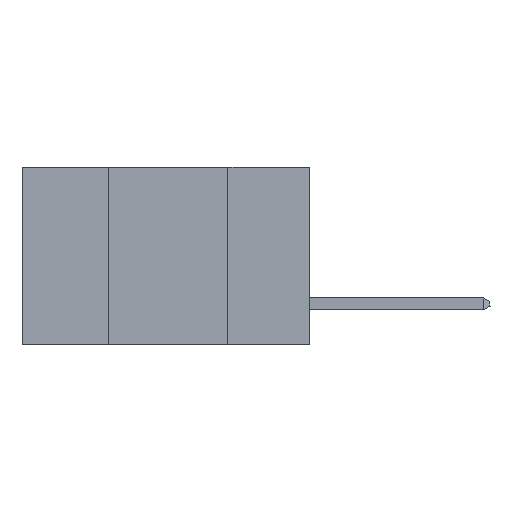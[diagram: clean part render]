
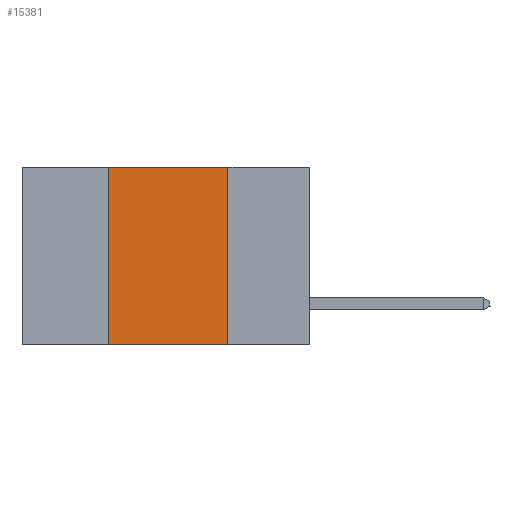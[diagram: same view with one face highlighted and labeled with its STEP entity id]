
A CAD part, left-side view. The second image highlights one B-rep face of the part: STEP entity #15381.
In plain terms, the highlighted planar face has unit normal (-1, 0, 0).
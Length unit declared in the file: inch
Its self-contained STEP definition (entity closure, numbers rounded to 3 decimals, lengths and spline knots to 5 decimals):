
#350 = FACE_OUTER_BOUND ( 'NONE', #20700, .T. ) ;
#760 = CARTESIAN_POINT ( 'NONE',  ( 0., 0.6, 0. ) ) ;
#2174 = ORIENTED_EDGE ( 'NONE', *, *, #10866, .F. ) ;
#2645 = DIRECTION ( 'NONE',  ( 0., 0., -1. ) ) ;
#2776 = DIRECTION ( 'NONE',  ( 0., 0., 1. ) ) ;
#3303 = VERTEX_POINT ( 'NONE', #8336 ) ;
#4249 = ORIENTED_EDGE ( 'NONE', *, *, #22775, .T. ) ;
#4461 = CARTESIAN_POINT ( 'NONE',  ( 0., 0.42, 0. ) ) ;
#4538 = ORIENTED_EDGE ( 'NONE', *, *, #21498, .F. ) ;
#5998 = DIRECTION ( 'NONE',  ( 0., -1., 0. ) ) ;
#7564 = DIRECTION ( 'NONE',  ( 1., 0., 0. ) ) ;
#8336 = CARTESIAN_POINT ( 'NONE',  ( 0., 0.42, -0.37 ) ) ;
#8653 = VECTOR ( 'NONE', #16114, 39.37008 ) ;
#9293 = PLANE ( 'NONE',  #10656 ) ;
#9879 = CARTESIAN_POINT ( 'NONE',  ( 0., 0.42, 0. ) ) ;
#9898 = CARTESIAN_POINT ( 'NONE',  ( 0., 0.17, 0. ) ) ;
#10656 = AXIS2_PLACEMENT_3D ( 'NONE', #760, #7564, #22130 ) ;
#10658 = LINE ( 'NONE', #11289, #13720 ) ;
#10866 = EDGE_CURVE ( 'NONE', #3303, #11276, #21980, .T. ) ;
#11249 = VECTOR ( 'NONE', #2645, 39.37008 ) ;
#11276 = VERTEX_POINT ( 'NONE', #4461 ) ;
#11289 = CARTESIAN_POINT ( 'NONE',  ( 0., 0.6, 0. ) ) ;
#11671 = VECTOR ( 'NONE', #2776, 39.37008 ) ;
#12108 = VERTEX_POINT ( 'NONE', #13793 ) ;
#13132 = VERTEX_POINT ( 'NONE', #21974 ) ;
#13326 = ORIENTED_EDGE ( 'NONE', *, *, #15401, .F. ) ;
#13720 = VECTOR ( 'NONE', #5998, 39.37008 ) ;
#13793 = CARTESIAN_POINT ( 'NONE',  ( 0., 0.17, 0. ) ) ;
#15381 = ADVANCED_FACE ( 'NONE', ( #350 ), #9293, .F. ) ;
#15401 = EDGE_CURVE ( 'NONE', #11276, #12108, #10658, .T. ) ;
#16114 = DIRECTION ( 'NONE',  ( 0., -1., 0. ) ) ;
#16196 = LINE ( 'NONE', #19590, #8653 ) ;
#19590 = CARTESIAN_POINT ( 'NONE',  ( 0., 0.6, -0.37 ) ) ;
#20145 = LINE ( 'NONE', #9898, #11249 ) ;
#20700 = EDGE_LOOP ( 'NONE', ( #4538, #13326, #2174, #4249 ) ) ;
#21498 = EDGE_CURVE ( 'NONE', #12108, #13132, #20145, .T. ) ;
#21974 = CARTESIAN_POINT ( 'NONE',  ( 0., 0.17, -0.37 ) ) ;
#21980 = LINE ( 'NONE', #9879, #11671 ) ;
#22130 = DIRECTION ( 'NONE',  ( 0., 0., -1. ) ) ;
#22775 = EDGE_CURVE ( 'NONE', #3303, #13132, #16196, .T. ) ;
